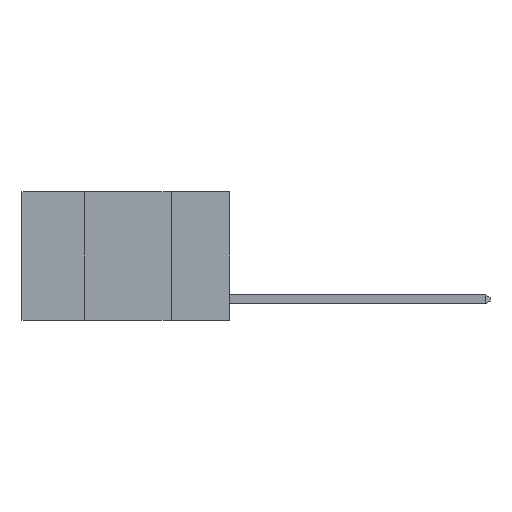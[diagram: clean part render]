
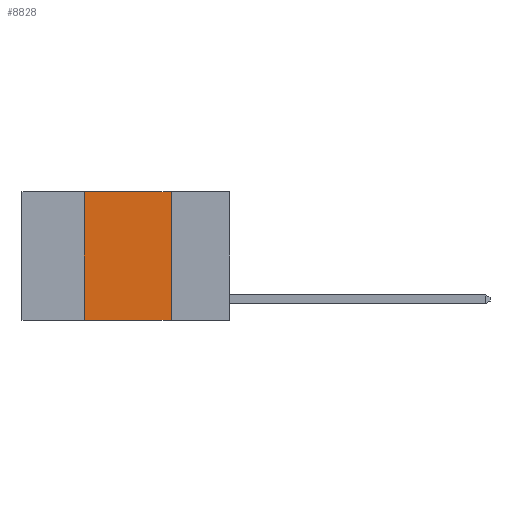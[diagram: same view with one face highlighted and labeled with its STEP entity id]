
A CAD part, left-side view. The second image highlights one B-rep face of the part: STEP entity #8828.
In plain terms, the highlighted planar face has unit normal (-1, 0, 0).
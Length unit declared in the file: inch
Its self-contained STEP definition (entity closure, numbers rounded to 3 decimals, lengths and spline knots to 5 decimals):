
#240 = AXIS2_PLACEMENT_3D ( 'NONE', #864, #3859, #9145 ) ;
#290 = EDGE_LOOP ( 'NONE', ( #6404, #9226, #9383, #8751 ) ) ;
#825 = LINE ( 'NONE', #2096, #4585 ) ;
#864 = CARTESIAN_POINT ( 'NONE',  ( 0., 0.6, 0. ) ) ;
#994 = DIRECTION ( 'NONE',  ( 0., -1., 0. ) ) ;
#1112 = FACE_OUTER_BOUND ( 'NONE', #290, .T. ) ;
#1172 = VECTOR ( 'NONE', #5760, 39.37008 ) ;
#1598 = CARTESIAN_POINT ( 'NONE',  ( 0., 0.17, 0. ) ) ;
#2056 = EDGE_CURVE ( 'NONE', #3798, #2098, #7081, .T. ) ;
#2096 = CARTESIAN_POINT ( 'NONE',  ( 0., 0.42, 0. ) ) ;
#2098 = VERTEX_POINT ( 'NONE', #3527 ) ;
#2353 = VERTEX_POINT ( 'NONE', #1598 ) ;
#2380 = PLANE ( 'NONE',  #240 ) ;
#2594 = EDGE_CURVE ( 'NONE', #3798, #9346, #825, .T. ) ;
#2909 = CARTESIAN_POINT ( 'NONE',  ( 0., 0.42, -0.37 ) ) ;
#2940 = CARTESIAN_POINT ( 'NONE',  ( 0., 0.42, 0. ) ) ;
#3394 = LINE ( 'NONE', #4997, #1172 ) ;
#3527 = CARTESIAN_POINT ( 'NONE',  ( 0., 0.17, -0.37 ) ) ;
#3798 = VERTEX_POINT ( 'NONE', #2909 ) ;
#3859 = DIRECTION ( 'NONE',  ( 1., 0., 0. ) ) ;
#4064 = LINE ( 'NONE', #5787, #5901 ) ;
#4505 = EDGE_CURVE ( 'NONE', #2353, #2098, #4064, .T. ) ;
#4585 = VECTOR ( 'NONE', #6081, 39.37008 ) ;
#4997 = CARTESIAN_POINT ( 'NONE',  ( 0., 0.6, 0. ) ) ;
#5089 = VECTOR ( 'NONE', #994, 39.37008 ) ;
#5520 = EDGE_CURVE ( 'NONE', #9346, #2353, #3394, .T. ) ;
#5760 = DIRECTION ( 'NONE',  ( 0., -1., 0. ) ) ;
#5787 = CARTESIAN_POINT ( 'NONE',  ( 0., 0.17, 0. ) ) ;
#5901 = VECTOR ( 'NONE', #6551, 39.37008 ) ;
#6081 = DIRECTION ( 'NONE',  ( 0., 0., 1. ) ) ;
#6404 = ORIENTED_EDGE ( 'NONE', *, *, #4505, .F. ) ;
#6551 = DIRECTION ( 'NONE',  ( 0., 0., -1. ) ) ;
#7081 = LINE ( 'NONE', #7487, #5089 ) ;
#7487 = CARTESIAN_POINT ( 'NONE',  ( 0., 0.6, -0.37 ) ) ;
#8751 = ORIENTED_EDGE ( 'NONE', *, *, #2056, .T. ) ;
#8828 = ADVANCED_FACE ( 'NONE', ( #1112 ), #2380, .F. ) ;
#9145 = DIRECTION ( 'NONE',  ( 0., 0., -1. ) ) ;
#9226 = ORIENTED_EDGE ( 'NONE', *, *, #5520, .F. ) ;
#9346 = VERTEX_POINT ( 'NONE', #2940 ) ;
#9383 = ORIENTED_EDGE ( 'NONE', *, *, #2594, .F. ) ;
